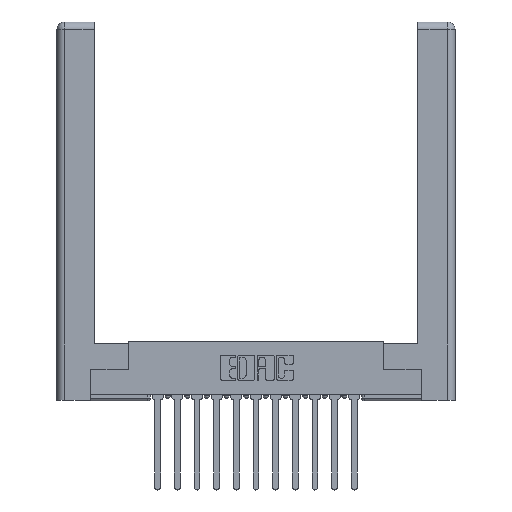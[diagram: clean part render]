
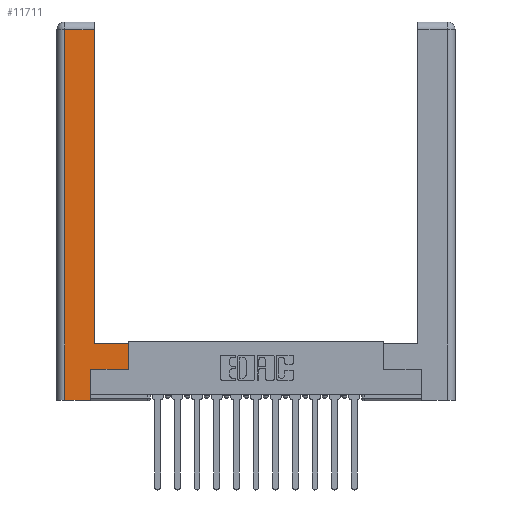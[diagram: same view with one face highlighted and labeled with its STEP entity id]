
A CAD part, top view. The second image highlights one B-rep face of the part: STEP entity #11711.
In plain terms, the highlighted planar face has unit normal (0, 0, 1).
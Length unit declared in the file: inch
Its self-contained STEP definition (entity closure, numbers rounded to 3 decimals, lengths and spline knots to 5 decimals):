
#151 = FACE_OUTER_BOUND ( 'NONE', #11375, .T. ) ;
#277 = VECTOR ( 'NONE', #2242, 39.37008 ) ;
#801 = LINE ( 'NONE', #10588, #11496 ) ;
#831 = CARTESIAN_POINT ( 'NONE',  ( 0.295, 0.45, 0. ) ) ;
#1293 = ORIENTED_EDGE ( 'NONE', *, *, #8253, .T. ) ;
#1708 = LINE ( 'NONE', #3864, #3788 ) ;
#1743 = ORIENTED_EDGE ( 'NONE', *, *, #14690, .T. ) ;
#1920 = VERTEX_POINT ( 'NONE', #831 ) ;
#2143 = CARTESIAN_POINT ( 'NONE',  ( 0.265, 0., 0. ) ) ;
#2242 = DIRECTION ( 'NONE',  ( 1., 0., 0. ) ) ;
#2554 = VECTOR ( 'NONE', #7532, 39.37008 ) ;
#3014 = DIRECTION ( 'NONE',  ( 0., 1., 0. ) ) ;
#3147 = VERTEX_POINT ( 'NONE', #3223 ) ;
#3223 = CARTESIAN_POINT ( 'NONE',  ( 0.295, 2.94, 0. ) ) ;
#3431 = DIRECTION ( 'NONE',  ( 0., -1., 0. ) ) ;
#3503 = LINE ( 'NONE', #4564, #277 ) ;
#3633 = VERTEX_POINT ( 'NONE', #14626 ) ;
#3718 = DIRECTION ( 'NONE',  ( -1., 0., 0. ) ) ;
#3788 = VECTOR ( 'NONE', #8862, 39.37008 ) ;
#3800 = VERTEX_POINT ( 'NONE', #8753 ) ;
#3864 = CARTESIAN_POINT ( 'NONE',  ( 0.295, 0.45, 0. ) ) ;
#4065 = LINE ( 'NONE', #11227, #2554 ) ;
#4312 = CARTESIAN_POINT ( 'NONE',  ( 0.0615, 0., 0. ) ) ;
#4380 = DIRECTION ( 'NONE',  ( 0., 1., 0. ) ) ;
#4408 = LINE ( 'NONE', #9321, #11925 ) ;
#4564 = CARTESIAN_POINT ( 'NONE',  ( 0.265, 0., 0. ) ) ;
#4964 = EDGE_CURVE ( 'NONE', #6135, #3800, #4065, .T. ) ;
#5289 = ORIENTED_EDGE ( 'NONE', *, *, #9542, .T. ) ;
#5427 = CARTESIAN_POINT ( 'NONE',  ( 0.295, 3., 0. ) ) ;
#5482 = VERTEX_POINT ( 'NONE', #15082 ) ;
#5700 = EDGE_CURVE ( 'NONE', #3633, #1920, #1708, .T. ) ;
#5811 = VECTOR ( 'NONE', #4380, 39.37008 ) ;
#6135 = VERTEX_POINT ( 'NONE', #13809 ) ;
#6267 = VERTEX_POINT ( 'NONE', #4312 ) ;
#6315 = DIRECTION ( 'NONE',  ( 0., 0., -1. ) ) ;
#6504 = VECTOR ( 'NONE', #3718, 39.37008 ) ;
#7270 = LINE ( 'NONE', #12168, #6504 ) ;
#7532 = DIRECTION ( 'NONE',  ( 1., 0., 0. ) ) ;
#7616 = AXIS2_PLACEMENT_3D ( 'NONE', #13784, #6315, #12581 ) ;
#8253 = EDGE_CURVE ( 'NONE', #3147, #5482, #7270, .T. ) ;
#8469 = ORIENTED_EDGE ( 'NONE', *, *, #5700, .T. ) ;
#8753 = CARTESIAN_POINT ( 'NONE',  ( 0.565, 0.245, 0. ) ) ;
#8862 = DIRECTION ( 'NONE',  ( -1., 0., 0. ) ) ;
#9321 = CARTESIAN_POINT ( 'NONE',  ( 0.0615, 0., 0. ) ) ;
#9542 = EDGE_CURVE ( 'NONE', #5482, #6267, #4408, .T. ) ;
#10251 = LINE ( 'NONE', #13949, #12281 ) ;
#10355 = ORIENTED_EDGE ( 'NONE', *, *, #12967, .T. ) ;
#10588 = CARTESIAN_POINT ( 'NONE',  ( 0.565, 0.45, 0. ) ) ;
#11227 = CARTESIAN_POINT ( 'NONE',  ( 0.565, 0.245, 0. ) ) ;
#11291 = PLANE ( 'NONE',  #7616 ) ;
#11375 = EDGE_LOOP ( 'NONE', ( #10355, #1293, #5289, #13139, #1743, #13569, #13834, #8469 ) ) ;
#11496 = VECTOR ( 'NONE', #15502, 39.37008 ) ;
#11711 = ADVANCED_FACE ( 'NONE', ( #151 ), #11291, .F. ) ;
#11925 = VECTOR ( 'NONE', #3431, 39.37008 ) ;
#12168 = CARTESIAN_POINT ( 'NONE',  ( 0.0615, 2.94, 0. ) ) ;
#12281 = VECTOR ( 'NONE', #3014, 39.37008 ) ;
#12581 = DIRECTION ( 'NONE',  ( -1., 0., 0. ) ) ;
#12820 = LINE ( 'NONE', #5427, #5811 ) ;
#12967 = EDGE_CURVE ( 'NONE', #1920, #3147, #12820, .T. ) ;
#13139 = ORIENTED_EDGE ( 'NONE', *, *, #15668, .T. ) ;
#13569 = ORIENTED_EDGE ( 'NONE', *, *, #4964, .T. ) ;
#13784 = CARTESIAN_POINT ( 'NONE',  ( 0., 0., 0. ) ) ;
#13809 = CARTESIAN_POINT ( 'NONE',  ( 0.265, 0.245, 0. ) ) ;
#13834 = ORIENTED_EDGE ( 'NONE', *, *, #14314, .T. ) ;
#13949 = CARTESIAN_POINT ( 'NONE',  ( 0.265, 0.245, 0. ) ) ;
#14314 = EDGE_CURVE ( 'NONE', #3800, #3633, #801, .T. ) ;
#14626 = CARTESIAN_POINT ( 'NONE',  ( 0.565, 0.45, 0. ) ) ;
#14690 = EDGE_CURVE ( 'NONE', #14761, #6135, #10251, .T. ) ;
#14761 = VERTEX_POINT ( 'NONE', #2143 ) ;
#15082 = CARTESIAN_POINT ( 'NONE',  ( 0.0615, 2.94, 0. ) ) ;
#15502 = DIRECTION ( 'NONE',  ( 0., 1., 0. ) ) ;
#15668 = EDGE_CURVE ( 'NONE', #6267, #14761, #3503, .T. ) ;
